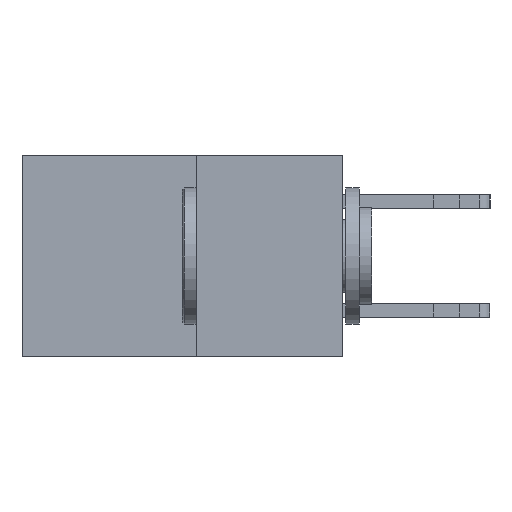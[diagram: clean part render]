
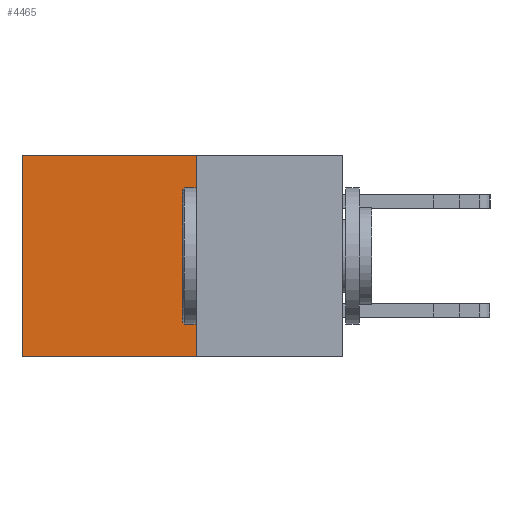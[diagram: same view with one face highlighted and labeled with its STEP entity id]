
A CAD part, left-side view. The second image highlights one B-rep face of the part: STEP entity #4465.
In plain terms, the highlighted planar face has unit normal (-1, 0, 0).
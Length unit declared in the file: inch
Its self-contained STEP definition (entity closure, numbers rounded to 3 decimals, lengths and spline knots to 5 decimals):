
#271 = FACE_OUTER_BOUND ( 'NONE', #12256, .T. ) ;
#330 = LINE ( 'NONE', #15686, #10373 ) ;
#910 = CARTESIAN_POINT ( 'NONE',  ( 0.277, 0.59, -0.37 ) ) ;
#2371 = CARTESIAN_POINT ( 'NONE',  ( 0.277, 0.59, 0. ) ) ;
#2445 = LINE ( 'NONE', #8899, #2864 ) ;
#2864 = VECTOR ( 'NONE', #9330, 39.37008 ) ;
#2923 = EDGE_CURVE ( 'NONE', #7088, #11232, #2445, .T. ) ;
#3049 = CARTESIAN_POINT ( 'NONE',  ( 0.277, 0.27, 0. ) ) ;
#3866 = VECTOR ( 'NONE', #8998, 39.37008 ) ;
#4120 = VERTEX_POINT ( 'NONE', #2371 ) ;
#4465 = ADVANCED_FACE ( 'NONE', ( #271 ), #9225, .F. ) ;
#4811 = VERTEX_POINT ( 'NONE', #910 ) ;
#5381 = EDGE_CURVE ( 'NONE', #7088, #4120, #7311, .T. ) ;
#6269 = LINE ( 'NONE', #12530, #15977 ) ;
#7088 = VERTEX_POINT ( 'NONE', #3049 ) ;
#7311 = LINE ( 'NONE', #8983, #3866 ) ;
#7532 = CARTESIAN_POINT ( 'NONE',  ( 0.277, 0.27, -0.37 ) ) ;
#7980 = DIRECTION ( 'NONE',  ( 0., 0., -1. ) ) ;
#8260 = DIRECTION ( 'NONE',  ( 1., 0., 0. ) ) ;
#8899 = CARTESIAN_POINT ( 'NONE',  ( 0.277, 0.27, -0.37 ) ) ;
#8983 = CARTESIAN_POINT ( 'NONE',  ( 0.277, 0.27, 0. ) ) ;
#8998 = DIRECTION ( 'NONE',  ( 0., 1., 0. ) ) ;
#9156 = CARTESIAN_POINT ( 'NONE',  ( 0.277, 0.27, -0.37 ) ) ;
#9225 = PLANE ( 'NONE',  #11567 ) ;
#9330 = DIRECTION ( 'NONE',  ( 0., 0., -1. ) ) ;
#9411 = ORIENTED_EDGE ( 'NONE', *, *, #2923, .F. ) ;
#9771 = EDGE_CURVE ( 'NONE', #11232, #4811, #6269, .T. ) ;
#9979 = ORIENTED_EDGE ( 'NONE', *, *, #9771, .F. ) ;
#10022 = DIRECTION ( 'NONE',  ( 0., 1., 0. ) ) ;
#10373 = VECTOR ( 'NONE', #13126, 39.37008 ) ;
#11232 = VERTEX_POINT ( 'NONE', #7532 ) ;
#11325 = ORIENTED_EDGE ( 'NONE', *, *, #12896, .T. ) ;
#11567 = AXIS2_PLACEMENT_3D ( 'NONE', #9156, #8260, #7980 ) ;
#11745 = ORIENTED_EDGE ( 'NONE', *, *, #5381, .T. ) ;
#12256 = EDGE_LOOP ( 'NONE', ( #11325, #9979, #9411, #11745 ) ) ;
#12530 = CARTESIAN_POINT ( 'NONE',  ( 0.277, 0.27, -0.37 ) ) ;
#12896 = EDGE_CURVE ( 'NONE', #4120, #4811, #330, .T. ) ;
#13126 = DIRECTION ( 'NONE',  ( 0., 0., -1. ) ) ;
#15686 = CARTESIAN_POINT ( 'NONE',  ( 0.277, 0.59, -0.37 ) ) ;
#15977 = VECTOR ( 'NONE', #10022, 39.37008 ) ;
